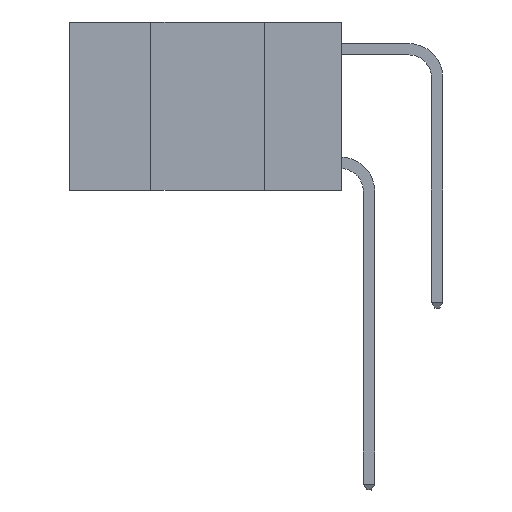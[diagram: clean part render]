
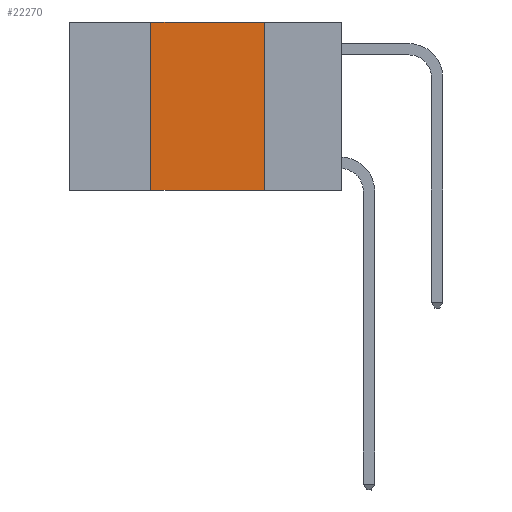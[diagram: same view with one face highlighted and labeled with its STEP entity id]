
A CAD part, left-side view. The second image highlights one B-rep face of the part: STEP entity #22270.
In plain terms, the highlighted planar face has unit normal (-1, 0, 0).
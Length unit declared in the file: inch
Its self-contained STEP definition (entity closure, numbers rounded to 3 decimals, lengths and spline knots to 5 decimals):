
#447 = DIRECTION ( 'NONE',  ( 1., 0., 0. ) ) ;
#877 = LINE ( 'NONE', #19893, #6707 ) ;
#910 = ORIENTED_EDGE ( 'NONE', *, *, #13475, .F. ) ;
#2356 = AXIS2_PLACEMENT_3D ( 'NONE', #21770, #447, #16832 ) ;
#3806 = CARTESIAN_POINT ( 'NONE',  ( 0., 0.17, 0. ) ) ;
#3860 = ORIENTED_EDGE ( 'NONE', *, *, #29749, .F. ) ;
#4095 = CARTESIAN_POINT ( 'NONE',  ( 0., 0.6, 0. ) ) ;
#4695 = DIRECTION ( 'NONE',  ( 0., -1., 0. ) ) ;
#5037 = DIRECTION ( 'NONE',  ( 0., 0., 1. ) ) ;
#6124 = CARTESIAN_POINT ( 'NONE',  ( 0., 0.17, -0.37 ) ) ;
#6707 = VECTOR ( 'NONE', #4695, 39.37008 ) ;
#7534 = LINE ( 'NONE', #9740, #19610 ) ;
#7827 = CARTESIAN_POINT ( 'NONE',  ( 0., 0.42, 0. ) ) ;
#7916 = PLANE ( 'NONE',  #2356 ) ;
#9740 = CARTESIAN_POINT ( 'NONE',  ( 0., 0.17, 0. ) ) ;
#11150 = VERTEX_POINT ( 'NONE', #16044 ) ;
#11307 = ORIENTED_EDGE ( 'NONE', *, *, #21630, .T. ) ;
#12495 = DIRECTION ( 'NONE',  ( 0., 0., -1. ) ) ;
#13475 = EDGE_CURVE ( 'NONE', #18497, #11150, #24179, .T. ) ;
#13580 = DIRECTION ( 'NONE',  ( 0., -1., 0. ) ) ;
#14386 = EDGE_LOOP ( 'NONE', ( #3860, #30278, #910, #11307 ) ) ;
#15402 = VERTEX_POINT ( 'NONE', #6124 ) ;
#15944 = LINE ( 'NONE', #4095, #20341 ) ;
#16044 = CARTESIAN_POINT ( 'NONE',  ( 0., 0.42, 0. ) ) ;
#16540 = CARTESIAN_POINT ( 'NONE',  ( 0., 0.42, -0.37 ) ) ;
#16832 = DIRECTION ( 'NONE',  ( 0., 0., -1. ) ) ;
#17288 = FACE_OUTER_BOUND ( 'NONE', #14386, .T. ) ;
#18497 = VERTEX_POINT ( 'NONE', #16540 ) ;
#19610 = VECTOR ( 'NONE', #12495, 39.37008 ) ;
#19893 = CARTESIAN_POINT ( 'NONE',  ( 0., 0.6, -0.37 ) ) ;
#20341 = VECTOR ( 'NONE', #13580, 39.37008 ) ;
#21630 = EDGE_CURVE ( 'NONE', #18497, #15402, #877, .T. ) ;
#21770 = CARTESIAN_POINT ( 'NONE',  ( 0., 0.6, 0. ) ) ;
#22270 = ADVANCED_FACE ( 'NONE', ( #17288 ), #7916, .F. ) ;
#24113 = VERTEX_POINT ( 'NONE', #3806 ) ;
#24179 = LINE ( 'NONE', #7827, #24632 ) ;
#24632 = VECTOR ( 'NONE', #5037, 39.37008 ) ;
#26077 = EDGE_CURVE ( 'NONE', #11150, #24113, #15944, .T. ) ;
#29749 = EDGE_CURVE ( 'NONE', #24113, #15402, #7534, .T. ) ;
#30278 = ORIENTED_EDGE ( 'NONE', *, *, #26077, .F. ) ;
